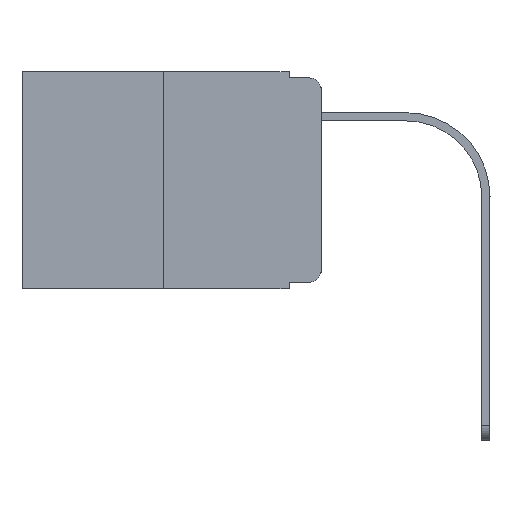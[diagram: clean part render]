
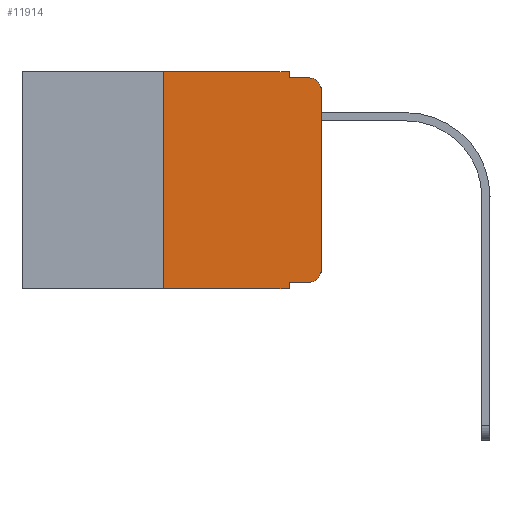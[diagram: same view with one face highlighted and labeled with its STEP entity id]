
A CAD part, left-side view. The second image highlights one B-rep face of the part: STEP entity #11914.
In plain terms, the highlighted planar face has unit normal (-1, 0, 0).
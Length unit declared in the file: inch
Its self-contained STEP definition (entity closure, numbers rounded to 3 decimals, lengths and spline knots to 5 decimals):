
#96 = DIRECTION ( 'NONE',  ( 0., 0., 1. ) ) ;
#242 = DIRECTION ( 'NONE',  ( 0., 0., -1. ) ) ;
#468 = VECTOR ( 'NONE', #8380, 39.37008 ) ;
#631 = DIRECTION ( 'NONE',  ( 0., -1., 0. ) ) ;
#959 = VECTOR ( 'NONE', #6811, 39.37008 ) ;
#1240 = DIRECTION ( 'NONE',  ( 1., 0., 0. ) ) ;
#1378 = EDGE_CURVE ( 'NONE', #4802, #6799, #8015, .T. ) ;
#1420 = EDGE_CURVE ( 'NONE', #9599, #2991, #2374, .T. ) ;
#1454 = ORIENTED_EDGE ( 'NONE', *, *, #9538, .F. ) ;
#1545 = CARTESIAN_POINT ( 'NONE',  ( 0., 0.051, 0. ) ) ;
#1978 = CARTESIAN_POINT ( 'NONE',  ( 0., 0.051, -0.333 ) ) ;
#2374 = CIRCLE ( 'NONE', #9146, 0.02 ) ;
#2799 = CARTESIAN_POINT ( 'NONE',  ( 0., 0.25, 0. ) ) ;
#2934 = ORIENTED_EDGE ( 'NONE', *, *, #1378, .F. ) ;
#2944 = AXIS2_PLACEMENT_3D ( 'NONE', #5000, #8670, #5860 ) ;
#2991 = VERTEX_POINT ( 'NONE', #8965 ) ;
#3564 = CARTESIAN_POINT ( 'NONE',  ( 0., 0.051, -0.01 ) ) ;
#3719 = VERTEX_POINT ( 'NONE', #8085 ) ;
#3723 = DIRECTION ( 'NONE',  ( 0., -1., 0. ) ) ;
#4160 = CARTESIAN_POINT ( 'NONE',  ( 0., 0.473, -0.343 ) ) ;
#4241 = ORIENTED_EDGE ( 'NONE', *, *, #11128, .T. ) ;
#4503 = EDGE_CURVE ( 'NONE', #2991, #3719, #4624, .T. ) ;
#4607 = CARTESIAN_POINT ( 'NONE',  ( 0., 0.02, -0.333 ) ) ;
#4624 = LINE ( 'NONE', #4807, #468 ) ;
#4696 = CARTESIAN_POINT ( 'NONE',  ( 0., 0.051, -0.333 ) ) ;
#4802 = VERTEX_POINT ( 'NONE', #8238 ) ;
#4807 = CARTESIAN_POINT ( 'NONE',  ( 0., 0., 0. ) ) ;
#4894 = VECTOR ( 'NONE', #3723, 39.37008 ) ;
#4969 = VECTOR ( 'NONE', #96, 39.37008 ) ;
#5000 = CARTESIAN_POINT ( 'NONE',  ( 0., 0.02, -0.03 ) ) ;
#5104 = CARTESIAN_POINT ( 'NONE',  ( 0., 0.473, 0. ) ) ;
#5860 = DIRECTION ( 'NONE',  ( 0., 0., -1. ) ) ;
#5902 = CARTESIAN_POINT ( 'NONE',  ( 0., 0.051, -0.01 ) ) ;
#6027 = EDGE_CURVE ( 'NONE', #6799, #6214, #11054, .T. ) ;
#6214 = VERTEX_POINT ( 'NONE', #9421 ) ;
#6279 = ORIENTED_EDGE ( 'NONE', *, *, #8302, .F. ) ;
#6799 = VERTEX_POINT ( 'NONE', #5902 ) ;
#6811 = DIRECTION ( 'NONE',  ( 0., -1., 0. ) ) ;
#7127 = EDGE_CURVE ( 'NONE', #10596, #9599, #10400, .T. ) ;
#7201 = CARTESIAN_POINT ( 'NONE',  ( 0., 0.02, -0.313 ) ) ;
#7469 = DIRECTION ( 'NONE',  ( 0., 0., -1. ) ) ;
#7523 = VECTOR ( 'NONE', #9842, 39.37008 ) ;
#7893 = ORIENTED_EDGE ( 'NONE', *, *, #12274, .T. ) ;
#8015 = LINE ( 'NONE', #8200, #11339 ) ;
#8085 = CARTESIAN_POINT ( 'NONE',  ( 0., 0., -0.03 ) ) ;
#8200 = CARTESIAN_POINT ( 'NONE',  ( 0., 0.051, 0. ) ) ;
#8228 = LINE ( 'NONE', #1545, #12336 ) ;
#8238 = CARTESIAN_POINT ( 'NONE',  ( 0., 0.051, 0. ) ) ;
#8282 = ORIENTED_EDGE ( 'NONE', *, *, #4503, .T. ) ;
#8302 = EDGE_CURVE ( 'NONE', #10596, #9807, #8228, .T. ) ;
#8380 = DIRECTION ( 'NONE',  ( 0., 0., 1. ) ) ;
#8505 = ORIENTED_EDGE ( 'NONE', *, *, #7127, .T. ) ;
#8519 = EDGE_CURVE ( 'NONE', #8905, #11951, #8648, .T. ) ;
#8648 = LINE ( 'NONE', #2799, #4969 ) ;
#8670 = DIRECTION ( 'NONE',  ( -1., 0., 0. ) ) ;
#8684 = CARTESIAN_POINT ( 'NONE',  ( 0., 0.473, 0. ) ) ;
#8905 = VERTEX_POINT ( 'NONE', #10391 ) ;
#8965 = CARTESIAN_POINT ( 'NONE',  ( 0., 0., -0.313 ) ) ;
#9097 = VECTOR ( 'NONE', #631, 39.37008 ) ;
#9118 = CIRCLE ( 'NONE', #2944, 0.02 ) ;
#9146 = AXIS2_PLACEMENT_3D ( 'NONE', #7201, #11877, #11071 ) ;
#9184 = EDGE_LOOP ( 'NONE', ( #8282, #4241, #11841, #2934, #1454, #10176, #7893, #6279, #8505, #9623 ) ) ;
#9421 = CARTESIAN_POINT ( 'NONE',  ( 0., 0.02, -0.01 ) ) ;
#9538 = EDGE_CURVE ( 'NONE', #11951, #4802, #9628, .T. ) ;
#9599 = VERTEX_POINT ( 'NONE', #4607 ) ;
#9623 = ORIENTED_EDGE ( 'NONE', *, *, #1420, .T. ) ;
#9628 = LINE ( 'NONE', #8684, #959 ) ;
#9807 = VERTEX_POINT ( 'NONE', #11599 ) ;
#9842 = DIRECTION ( 'NONE',  ( 0., -1., 0. ) ) ;
#10176 = ORIENTED_EDGE ( 'NONE', *, *, #8519, .F. ) ;
#10391 = CARTESIAN_POINT ( 'NONE',  ( 0., 0.25, -0.343 ) ) ;
#10400 = LINE ( 'NONE', #1978, #4894 ) ;
#10596 = VERTEX_POINT ( 'NONE', #4696 ) ;
#10912 = PLANE ( 'NONE',  #11145 ) ;
#11035 = CARTESIAN_POINT ( 'NONE',  ( 0., 0.25, 0. ) ) ;
#11054 = LINE ( 'NONE', #3564, #9097 ) ;
#11071 = DIRECTION ( 'NONE',  ( 0., 0., -1. ) ) ;
#11128 = EDGE_CURVE ( 'NONE', #3719, #6214, #9118, .T. ) ;
#11145 = AXIS2_PLACEMENT_3D ( 'NONE', #5104, #1240, #242 ) ;
#11339 = VECTOR ( 'NONE', #11818, 39.37008 ) ;
#11599 = CARTESIAN_POINT ( 'NONE',  ( 0., 0.051, -0.343 ) ) ;
#11711 = LINE ( 'NONE', #4160, #7523 ) ;
#11731 = FACE_OUTER_BOUND ( 'NONE', #9184, .T. ) ;
#11818 = DIRECTION ( 'NONE',  ( 0., 0., -1. ) ) ;
#11841 = ORIENTED_EDGE ( 'NONE', *, *, #6027, .F. ) ;
#11877 = DIRECTION ( 'NONE',  ( -1., 0., 0. ) ) ;
#11914 = ADVANCED_FACE ( 'NONE', ( #11731 ), #10912, .F. ) ;
#11951 = VERTEX_POINT ( 'NONE', #11035 ) ;
#12274 = EDGE_CURVE ( 'NONE', #8905, #9807, #11711, .T. ) ;
#12336 = VECTOR ( 'NONE', #7469, 39.37008 ) ;
